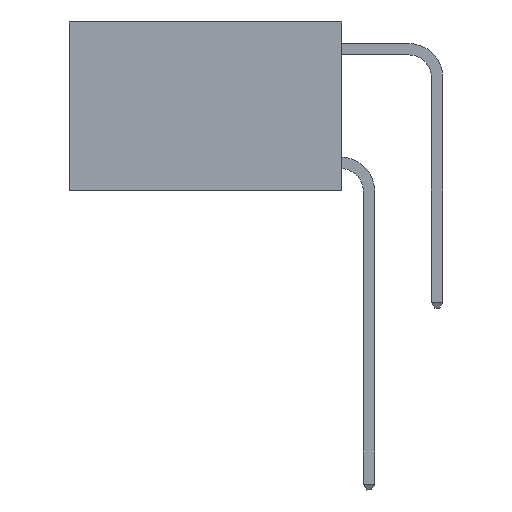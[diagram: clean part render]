
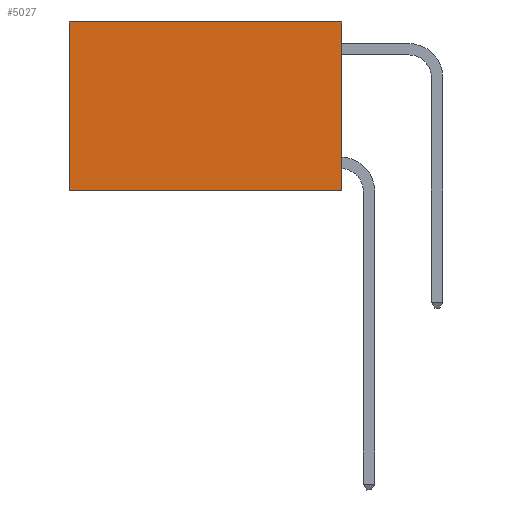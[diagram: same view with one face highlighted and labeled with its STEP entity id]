
A CAD part, left-side view. The second image highlights one B-rep face of the part: STEP entity #5027.
In plain terms, the highlighted planar face has unit normal (-1, 0, 0).
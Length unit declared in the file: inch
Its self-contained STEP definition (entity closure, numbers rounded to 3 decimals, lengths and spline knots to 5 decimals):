
#162 = ORIENTED_EDGE ( 'NONE', *, *, #10912, .F. ) ;
#1249 = VERTEX_POINT ( 'NONE', #4158 ) ;
#1262 = LINE ( 'NONE', #3525, #5810 ) ;
#1454 = EDGE_CURVE ( 'NONE', #1249, #8478, #1262, .T. ) ;
#1760 = LINE ( 'NONE', #9374, #3590 ) ;
#2109 = CARTESIAN_POINT ( 'NONE',  ( 0.2625, 0., 0. ) ) ;
#2113 = DIRECTION ( 'NONE',  ( 0., 0., -1. ) ) ;
#2504 = EDGE_CURVE ( 'NONE', #9211, #6793, #7314, .T. ) ;
#2593 = ORIENTED_EDGE ( 'NONE', *, *, #2504, .F. ) ;
#2800 = VECTOR ( 'NONE', #2113, 39.37008 ) ;
#3376 = CARTESIAN_POINT ( 'NONE',  ( 0.2625, 0.6, -0.37 ) ) ;
#3525 = CARTESIAN_POINT ( 'NONE',  ( 0.2625, 0.6, 0. ) ) ;
#3590 = VECTOR ( 'NONE', #4918, 39.37008 ) ;
#4013 = DIRECTION ( 'NONE',  ( 0., 0., -1. ) ) ;
#4158 = CARTESIAN_POINT ( 'NONE',  ( 0.2625, 0.6, 0. ) ) ;
#4739 = EDGE_LOOP ( 'NONE', ( #9464, #162, #2593, #7389 ) ) ;
#4918 = DIRECTION ( 'NONE',  ( 0., 1., 0. ) ) ;
#5027 = ADVANCED_FACE ( 'NONE', ( #10997 ), #11418, .F. ) ;
#5810 = VECTOR ( 'NONE', #4013, 39.37008 ) ;
#6793 = VERTEX_POINT ( 'NONE', #7033 ) ;
#7033 = CARTESIAN_POINT ( 'NONE',  ( 0.2625, 0., -0.37 ) ) ;
#7314 = LINE ( 'NONE', #2109, #2800 ) ;
#7389 = ORIENTED_EDGE ( 'NONE', *, *, #9835, .T. ) ;
#7841 = DIRECTION ( 'NONE',  ( 0., 1., 0. ) ) ;
#8261 = VECTOR ( 'NONE', #7841, 39.37008 ) ;
#8478 = VERTEX_POINT ( 'NONE', #3376 ) ;
#8542 = LINE ( 'NONE', #9615, #8261 ) ;
#9211 = VERTEX_POINT ( 'NONE', #11476 ) ;
#9341 = AXIS2_PLACEMENT_3D ( 'NONE', #11169, #11131, #11105 ) ;
#9374 = CARTESIAN_POINT ( 'NONE',  ( 0.2625, 0., -0.37 ) ) ;
#9464 = ORIENTED_EDGE ( 'NONE', *, *, #1454, .T. ) ;
#9615 = CARTESIAN_POINT ( 'NONE',  ( 0.2625, 0., 0. ) ) ;
#9835 = EDGE_CURVE ( 'NONE', #9211, #1249, #8542, .T. ) ;
#10912 = EDGE_CURVE ( 'NONE', #6793, #8478, #1760, .T. ) ;
#10997 = FACE_OUTER_BOUND ( 'NONE', #4739, .T. ) ;
#11105 = DIRECTION ( 'NONE',  ( 0., 0., -1. ) ) ;
#11131 = DIRECTION ( 'NONE',  ( 1., 0., 0. ) ) ;
#11169 = CARTESIAN_POINT ( 'NONE',  ( 0.2625, 0., 0. ) ) ;
#11418 = PLANE ( 'NONE',  #9341 ) ;
#11476 = CARTESIAN_POINT ( 'NONE',  ( 0.2625, 0., 0. ) ) ;
